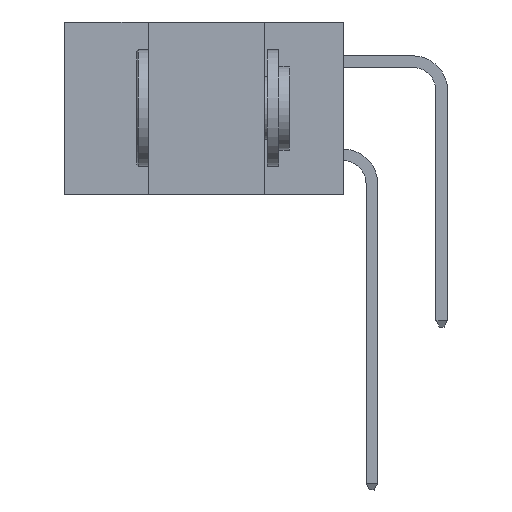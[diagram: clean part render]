
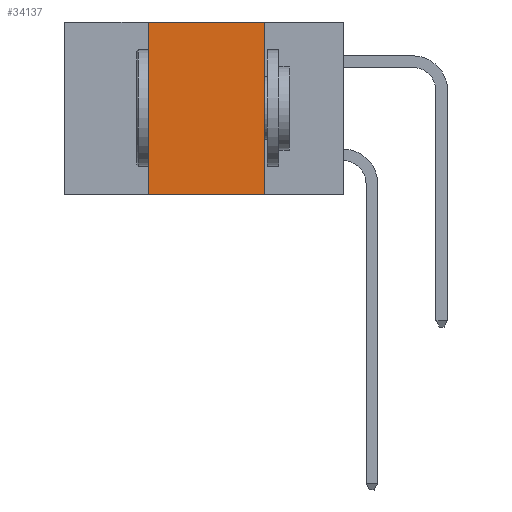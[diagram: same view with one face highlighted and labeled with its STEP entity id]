
A CAD part, left-side view. The second image highlights one B-rep face of the part: STEP entity #34137.
In plain terms, the highlighted planar face has unit normal (-1, 0, 0).
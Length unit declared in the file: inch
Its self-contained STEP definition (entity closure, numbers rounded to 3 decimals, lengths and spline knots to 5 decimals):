
#687 = CARTESIAN_POINT ( 'NONE',  ( 0., 0.17, 0. ) ) ;
#2819 = DIRECTION ( 'NONE',  ( 1., 0., 0. ) ) ;
#2834 = VERTEX_POINT ( 'NONE', #33456 ) ;
#5052 = CARTESIAN_POINT ( 'NONE',  ( 0., 0.17, -0.37 ) ) ;
#7522 = LINE ( 'NONE', #29065, #17279 ) ;
#8660 = AXIS2_PLACEMENT_3D ( 'NONE', #19569, #2819, #22382 ) ;
#8736 = DIRECTION ( 'NONE',  ( 0., 0., 1. ) ) ;
#8834 = CARTESIAN_POINT ( 'NONE',  ( 0., 0.6, 0. ) ) ;
#8855 = VERTEX_POINT ( 'NONE', #30504 ) ;
#9419 = VERTEX_POINT ( 'NONE', #5052 ) ;
#12738 = ORIENTED_EDGE ( 'NONE', *, *, #20734, .T. ) ;
#13336 = EDGE_CURVE ( 'NONE', #20516, #9419, #15703, .T. ) ;
#13478 = ORIENTED_EDGE ( 'NONE', *, *, #27943, .F. ) ;
#13826 = CARTESIAN_POINT ( 'NONE',  ( 0., 0.17, 0. ) ) ;
#14467 = ORIENTED_EDGE ( 'NONE', *, *, #17058, .F. ) ;
#15703 = LINE ( 'NONE', #687, #29426 ) ;
#16803 = PLANE ( 'NONE',  #8660 ) ;
#17058 = EDGE_CURVE ( 'NONE', #8855, #2834, #28065, .T. ) ;
#17279 = VECTOR ( 'NONE', #20921, 39.37008 ) ;
#19569 = CARTESIAN_POINT ( 'NONE',  ( 0., 0.6, 0. ) ) ;
#20516 = VERTEX_POINT ( 'NONE', #13826 ) ;
#20734 = EDGE_CURVE ( 'NONE', #8855, #9419, #7522, .T. ) ;
#20777 = VECTOR ( 'NONE', #8736, 39.37008 ) ;
#20921 = DIRECTION ( 'NONE',  ( 0., -1., 0. ) ) ;
#22382 = DIRECTION ( 'NONE',  ( 0., 0., -1. ) ) ;
#23186 = DIRECTION ( 'NONE',  ( 0., 0., -1. ) ) ;
#24181 = VECTOR ( 'NONE', #28218, 39.37008 ) ;
#25171 = CARTESIAN_POINT ( 'NONE',  ( 0., 0.42, 0. ) ) ;
#27943 = EDGE_CURVE ( 'NONE', #2834, #20516, #31413, .T. ) ;
#28065 = LINE ( 'NONE', #25171, #20777 ) ;
#28218 = DIRECTION ( 'NONE',  ( 0., -1., 0. ) ) ;
#29065 = CARTESIAN_POINT ( 'NONE',  ( 0., 0.6, -0.37 ) ) ;
#29426 = VECTOR ( 'NONE', #23186, 39.37008 ) ;
#30504 = CARTESIAN_POINT ( 'NONE',  ( 0., 0.42, -0.37 ) ) ;
#31298 = EDGE_LOOP ( 'NONE', ( #31323, #13478, #14467, #12738 ) ) ;
#31323 = ORIENTED_EDGE ( 'NONE', *, *, #13336, .F. ) ;
#31413 = LINE ( 'NONE', #8834, #24181 ) ;
#33456 = CARTESIAN_POINT ( 'NONE',  ( 0., 0.42, 0. ) ) ;
#34137 = ADVANCED_FACE ( 'NONE', ( #35469 ), #16803, .F. ) ;
#35469 = FACE_OUTER_BOUND ( 'NONE', #31298, .T. ) ;
